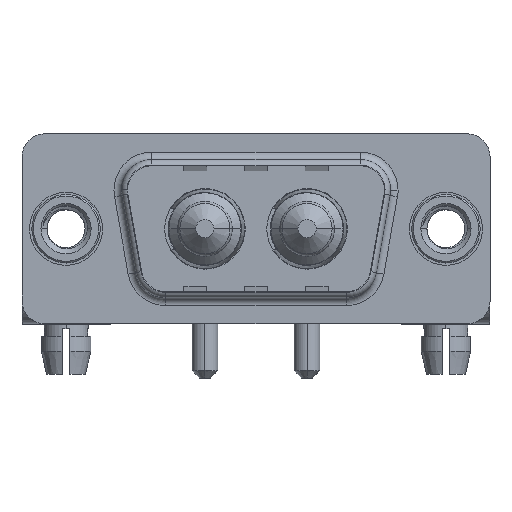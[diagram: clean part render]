
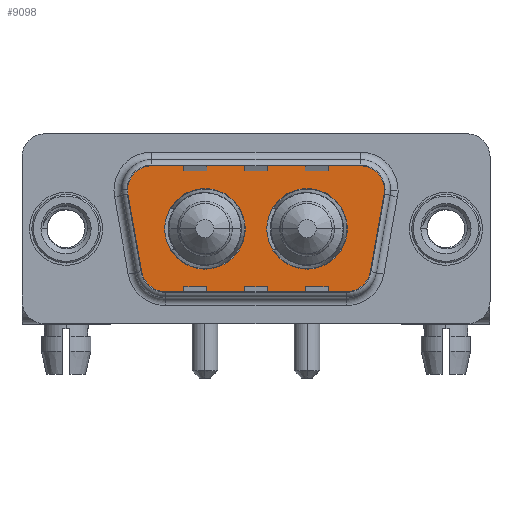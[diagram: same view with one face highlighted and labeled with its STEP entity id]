
A CAD part, top view. The second image highlights one B-rep face of the part: STEP entity #9098.
In plain terms, the highlighted planar face has unit normal (0, 0, 1).
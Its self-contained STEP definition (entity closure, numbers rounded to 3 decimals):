
#83 = CIRCLE ( 'NONE', #9196, 2. ) ;
#228 = DIRECTION ( 'NONE',  ( 1., 0., 0. ) ) ;
#256 = DIRECTION ( 'NONE',  ( 0., 0., 1. ) ) ;
#387 = CARTESIAN_POINT ( 'NONE',  ( 6.459, -4.9, 0. ) ) ;
#760 = CARTESIAN_POINT ( 'NONE',  ( 15.86, 0., 0. ) ) ;
#762 = DIRECTION ( 'NONE',  ( -1., 0., 0. ) ) ;
#965 = FACE_BOUND ( 'NONE', #14018, .T. ) ;
#1153 = ORIENTED_EDGE ( 'NONE', *, *, #8143, .T. ) ;
#1170 = VECTOR ( 'NONE', #9707, 1000. ) ;
#1559 = CIRCLE ( 'NONE', #7395, 2. ) ;
#1815 = CARTESIAN_POINT ( 'NONE',  ( 21.564, 2.9, 0. ) ) ;
#1910 = CARTESIAN_POINT ( 'NONE',  ( 18.541, -2.9, 0. ) ) ;
#1963 = VERTEX_POINT ( 'NONE', #14631 ) ;
#1988 = LINE ( 'NONE', #7792, #9951 ) ;
#2006 = CIRCLE ( 'NONE', #7332, 2.65 ) ;
#2370 = CIRCLE ( 'NONE', #6185, 2.65 ) ;
#2403 = CARTESIAN_POINT ( 'NONE',  ( 13.21, 0., 0. ) ) ;
#2679 = VERTEX_POINT ( 'NONE', #1815 ) ;
#2831 = DIRECTION ( 'NONE',  ( -1., 0., 0. ) ) ;
#2948 = CIRCLE ( 'NONE', #12589, 2.65 ) ;
#2974 = DIRECTION ( 'NONE',  ( 0., 0., 1. ) ) ;
#3051 = CARTESIAN_POINT ( 'NONE',  ( 5.436, 2.9, 0. ) ) ;
#3069 = EDGE_CURVE ( 'NONE', #4582, #2679, #11904, .T. ) ;
#3158 = AXIS2_PLACEMENT_3D ( 'NONE', #5459, #9091, #15057 ) ;
#3289 = VECTOR ( 'NONE', #2831, 1000. ) ;
#3340 = CARTESIAN_POINT ( 'NONE',  ( 18.541, -4.9, 0. ) ) ;
#3460 = ORIENTED_EDGE ( 'NONE', *, *, #10264, .F. ) ;
#3563 = DIRECTION ( 'NONE',  ( 1., 0., 0. ) ) ;
#3587 = DIRECTION ( 'NONE',  ( 1., 0., 0. ) ) ;
#3810 = VERTEX_POINT ( 'NONE', #10971 ) ;
#4001 = DIRECTION ( 'NONE',  ( 1., 0., 0. ) ) ;
#4027 = LINE ( 'NONE', #14907, #3289 ) ;
#4058 = VERTEX_POINT ( 'NONE', #7776 ) ;
#4127 = CARTESIAN_POINT ( 'NONE',  ( 6.459, -2.9, 0. ) ) ;
#4176 = ORIENTED_EDGE ( 'NONE', *, *, #10462, .T. ) ;
#4518 = ORIENTED_EDGE ( 'NONE', *, *, #6807, .F. ) ;
#4582 = VERTEX_POINT ( 'NONE', #10975 ) ;
#4627 = CARTESIAN_POINT ( 'NONE',  ( 5.436, 4.9, 0. ) ) ;
#4873 = CARTESIAN_POINT ( 'NONE',  ( 3.466, 2.553, 0. ) ) ;
#5382 = ORIENTED_EDGE ( 'NONE', *, *, #15604, .T. ) ;
#5415 = ORIENTED_EDGE ( 'NONE', *, *, #13602, .T. ) ;
#5421 = EDGE_CURVE ( 'NONE', #10006, #15214, #1559, .T. ) ;
#5459 = CARTESIAN_POINT ( 'NONE',  ( 19.564, 2.9, 0. ) ) ;
#5774 = VECTOR ( 'NONE', #228, 1000. ) ;
#5807 = CARTESIAN_POINT ( 'NONE',  ( 18.541, -2.9, 0. ) ) ;
#6105 = CARTESIAN_POINT ( 'NONE',  ( 9.14, 0., 0. ) ) ;
#6170 = AXIS2_PLACEMENT_3D ( 'NONE', #6540, #7578, #4001 ) ;
#6185 = AXIS2_PLACEMENT_3D ( 'NONE', #6105, #7380, #3563 ) ;
#6540 = CARTESIAN_POINT ( 'NONE',  ( 9.14, 0., 0. ) ) ;
#6691 = VERTEX_POINT ( 'NONE', #7590 ) ;
#6714 = DIRECTION ( 'NONE',  ( 1., 0., 0. ) ) ;
#6807 = EDGE_CURVE ( 'NONE', #6691, #8392, #2948, .T. ) ;
#7071 = EDGE_CURVE ( 'NONE', #15214, #9743, #15591, .T. ) ;
#7332 = AXIS2_PLACEMENT_3D ( 'NONE', #9623, #256, #3587 ) ;
#7380 = DIRECTION ( 'NONE',  ( 0., 0., 1. ) ) ;
#7395 = AXIS2_PLACEMENT_3D ( 'NONE', #3051, #2974, #6714 ) ;
#7396 = CARTESIAN_POINT ( 'NONE',  ( 6.459, -4.9, 0. ) ) ;
#7578 = DIRECTION ( 'NONE',  ( 0., 0., 1. ) ) ;
#7590 = CARTESIAN_POINT ( 'NONE',  ( 18.51, 0., 0. ) ) ;
#7776 = CARTESIAN_POINT ( 'NONE',  ( 19.564, 4.9, 0. ) ) ;
#7786 = EDGE_LOOP ( 'NONE', ( #4176, #5415, #10445, #1153, #8497, #15259, #9658, #9423, #5382 ) ) ;
#7792 = CARTESIAN_POINT ( 'NONE',  ( 21.534, 2.553, 0. ) ) ;
#7906 = EDGE_LOOP ( 'NONE', ( #4518, #3460 ) ) ;
#8023 = DIRECTION ( 'NONE',  ( 0., 0., 1. ) ) ;
#8143 = EDGE_CURVE ( 'NONE', #2679, #4058, #14524, .T. ) ;
#8178 = CARTESIAN_POINT ( 'NONE',  ( 3.466, 2.553, 0. ) ) ;
#8392 = VERTEX_POINT ( 'NONE', #2403 ) ;
#8497 = ORIENTED_EDGE ( 'NONE', *, *, #10680, .T. ) ;
#8512 = EDGE_CURVE ( 'NONE', #1963, #3810, #15561, .T. ) ;
#9029 = ORIENTED_EDGE ( 'NONE', *, *, #8512, .F. ) ;
#9091 = DIRECTION ( 'NONE',  ( 0., 0., 1. ) ) ;
#9098 = ADVANCED_FACE ( 'NONE', ( #12790, #965, #15481 ), #11680, .T. ) ;
#9196 = AXIS2_PLACEMENT_3D ( 'NONE', #4127, #12865, #15168 ) ;
#9203 = EDGE_CURVE ( 'NONE', #3810, #1963, #2370, .T. ) ;
#9374 = AXIS2_PLACEMENT_3D ( 'NONE', #1910, #14299, #10642 ) ;
#9423 = ORIENTED_EDGE ( 'NONE', *, *, #12601, .T. ) ;
#9623 = CARTESIAN_POINT ( 'NONE',  ( 15.86, 0., 0. ) ) ;
#9658 = ORIENTED_EDGE ( 'NONE', *, *, #7071, .T. ) ;
#9707 = DIRECTION ( 'NONE',  ( 0.174, -0.985, 0. ) ) ;
#9743 = VERTEX_POINT ( 'NONE', #9873 ) ;
#9873 = CARTESIAN_POINT ( 'NONE',  ( 4.489, -3.247, 0. ) ) ;
#9951 = VECTOR ( 'NONE', #12636, 1000. ) ;
#10006 = VERTEX_POINT ( 'NONE', #4627 ) ;
#10130 = CIRCLE ( 'NONE', #9374, 2. ) ;
#10201 = CARTESIAN_POINT ( 'NONE',  ( 19.564, 2.9, 0. ) ) ;
#10264 = EDGE_CURVE ( 'NONE', #8392, #6691, #2006, .T. ) ;
#10445 = ORIENTED_EDGE ( 'NONE', *, *, #3069, .T. ) ;
#10462 = EDGE_CURVE ( 'NONE', #13714, #12916, #10130, .T. ) ;
#10474 = DIRECTION ( 'NONE',  ( 1., 0., 0. ) ) ;
#10642 = DIRECTION ( 'NONE',  ( 1., 0., 0. ) ) ;
#10680 = EDGE_CURVE ( 'NONE', #4058, #10006, #4027, .T. ) ;
#10971 = CARTESIAN_POINT ( 'NONE',  ( 6.49, 0., 0. ) ) ;
#10975 = CARTESIAN_POINT ( 'NONE',  ( 21.534, 2.553, 0. ) ) ;
#11002 = VERTEX_POINT ( 'NONE', #7396 ) ;
#11680 = PLANE ( 'NONE',  #15061 ) ;
#11873 = DIRECTION ( 'NONE',  ( 0., 0., 1. ) ) ;
#11904 = CIRCLE ( 'NONE', #3158, 2. ) ;
#12589 = AXIS2_PLACEMENT_3D ( 'NONE', #760, #11873, #12824 ) ;
#12601 = EDGE_CURVE ( 'NONE', #9743, #11002, #83, .T. ) ;
#12636 = DIRECTION ( 'NONE',  ( 0.174, 0.985, 0. ) ) ;
#12790 = FACE_BOUND ( 'NONE', #7906, .T. ) ;
#12824 = DIRECTION ( 'NONE',  ( 1., 0., 0. ) ) ;
#12865 = DIRECTION ( 'NONE',  ( 0., 0., 1. ) ) ;
#12916 = VERTEX_POINT ( 'NONE', #15686 ) ;
#13602 = EDGE_CURVE ( 'NONE', #12916, #4582, #1988, .T. ) ;
#13714 = VERTEX_POINT ( 'NONE', #3340 ) ;
#13798 = ORIENTED_EDGE ( 'NONE', *, *, #9203, .F. ) ;
#14018 = EDGE_LOOP ( 'NONE', ( #9029, #13798 ) ) ;
#14299 = DIRECTION ( 'NONE',  ( 0., 0., 1. ) ) ;
#14524 = CIRCLE ( 'NONE', #14785, 2. ) ;
#14631 = CARTESIAN_POINT ( 'NONE',  ( 11.79, 0., 0. ) ) ;
#14785 = AXIS2_PLACEMENT_3D ( 'NONE', #10201, #15047, #762 ) ;
#14838 = LINE ( 'NONE', #387, #5774 ) ;
#14907 = CARTESIAN_POINT ( 'NONE',  ( 5.436, 4.9, 0. ) ) ;
#15047 = DIRECTION ( 'NONE',  ( 0., 0., 1. ) ) ;
#15057 = DIRECTION ( 'NONE',  ( -1., 0., 0. ) ) ;
#15061 = AXIS2_PLACEMENT_3D ( 'NONE', #5807, #8023, #10474 ) ;
#15168 = DIRECTION ( 'NONE',  ( -1., 0., 0. ) ) ;
#15214 = VERTEX_POINT ( 'NONE', #8178 ) ;
#15259 = ORIENTED_EDGE ( 'NONE', *, *, #5421, .T. ) ;
#15481 = FACE_OUTER_BOUND ( 'NONE', #7786, .T. ) ;
#15561 = CIRCLE ( 'NONE', #6170, 2.65 ) ;
#15591 = LINE ( 'NONE', #4873, #1170 ) ;
#15604 = EDGE_CURVE ( 'NONE', #11002, #13714, #14838, .T. ) ;
#15686 = CARTESIAN_POINT ( 'NONE',  ( 20.511, -3.247, 0. ) ) ;
